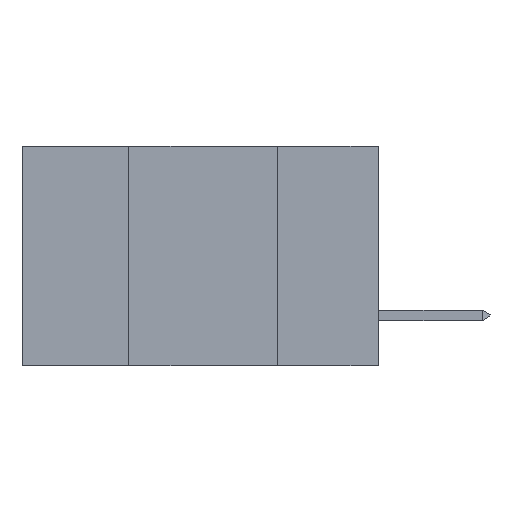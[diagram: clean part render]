
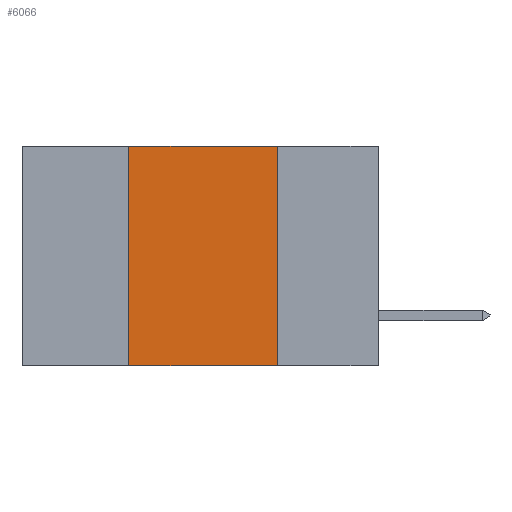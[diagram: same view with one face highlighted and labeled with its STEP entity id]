
A CAD part, left-side view. The second image highlights one B-rep face of the part: STEP entity #6066.
In plain terms, the highlighted planar face has unit normal (-1, 0, 0).
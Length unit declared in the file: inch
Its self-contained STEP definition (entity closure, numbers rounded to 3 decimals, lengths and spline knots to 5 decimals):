
#227 = CARTESIAN_POINT ( 'NONE',  ( 0., 0.42, -0.37 ) ) ;
#1244 = CARTESIAN_POINT ( 'NONE',  ( 0., 0.42, 0. ) ) ;
#1372 = FACE_OUTER_BOUND ( 'NONE', #9336, .T. ) ;
#1496 = LINE ( 'NONE', #2828, #10437 ) ;
#2828 = CARTESIAN_POINT ( 'NONE',  ( 0., 0.6, 0. ) ) ;
#2936 = CARTESIAN_POINT ( 'NONE',  ( 0., 0.17, 0. ) ) ;
#3825 = LINE ( 'NONE', #8459, #8410 ) ;
#3957 = EDGE_CURVE ( 'NONE', #4776, #8018, #7815, .T. ) ;
#4419 = ORIENTED_EDGE ( 'NONE', *, *, #3957, .T. ) ;
#4710 = LINE ( 'NONE', #10534, #7535 ) ;
#4776 = VERTEX_POINT ( 'NONE', #227 ) ;
#5010 = ORIENTED_EDGE ( 'NONE', *, *, #6257, .F. ) ;
#5046 = DIRECTION ( 'NONE',  ( 0., 0., -1. ) ) ;
#5150 = CARTESIAN_POINT ( 'NONE',  ( 0., 0.6, 0. ) ) ;
#5184 = AXIS2_PLACEMENT_3D ( 'NONE', #5150, #9263, #5046 ) ;
#5288 = EDGE_CURVE ( 'NONE', #4776, #5375, #4710, .T. ) ;
#5375 = VERTEX_POINT ( 'NONE', #1244 ) ;
#5844 = VECTOR ( 'NONE', #7153, 39.37008 ) ;
#6066 = ADVANCED_FACE ( 'NONE', ( #1372 ), #6768, .F. ) ;
#6257 = EDGE_CURVE ( 'NONE', #5375, #10219, #1496, .T. ) ;
#6466 = CARTESIAN_POINT ( 'NONE',  ( 0., 0.6, -0.37 ) ) ;
#6565 = CARTESIAN_POINT ( 'NONE',  ( 0., 0.17, -0.37 ) ) ;
#6768 = PLANE ( 'NONE',  #5184 ) ;
#7153 = DIRECTION ( 'NONE',  ( 0., -1., 0. ) ) ;
#7259 = ORIENTED_EDGE ( 'NONE', *, *, #7721, .F. ) ;
#7535 = VECTOR ( 'NONE', #9662, 39.37008 ) ;
#7721 = EDGE_CURVE ( 'NONE', #10219, #8018, #3825, .T. ) ;
#7815 = LINE ( 'NONE', #6466, #5844 ) ;
#8018 = VERTEX_POINT ( 'NONE', #6565 ) ;
#8053 = DIRECTION ( 'NONE',  ( 0., -1., 0. ) ) ;
#8410 = VECTOR ( 'NONE', #8502, 39.37008 ) ;
#8459 = CARTESIAN_POINT ( 'NONE',  ( 0., 0.17, 0. ) ) ;
#8502 = DIRECTION ( 'NONE',  ( 0., 0., -1. ) ) ;
#9263 = DIRECTION ( 'NONE',  ( 1., 0., 0. ) ) ;
#9336 = EDGE_LOOP ( 'NONE', ( #7259, #5010, #11187, #4419 ) ) ;
#9662 = DIRECTION ( 'NONE',  ( 0., 0., 1. ) ) ;
#10219 = VERTEX_POINT ( 'NONE', #2936 ) ;
#10437 = VECTOR ( 'NONE', #8053, 39.37008 ) ;
#10534 = CARTESIAN_POINT ( 'NONE',  ( 0., 0.42, 0. ) ) ;
#11187 = ORIENTED_EDGE ( 'NONE', *, *, #5288, .F. ) ;
